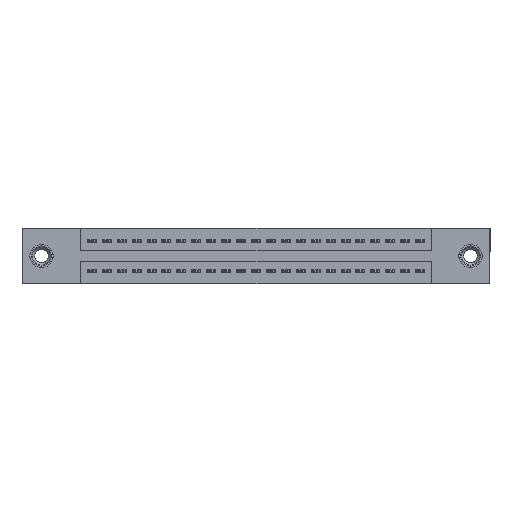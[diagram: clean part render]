
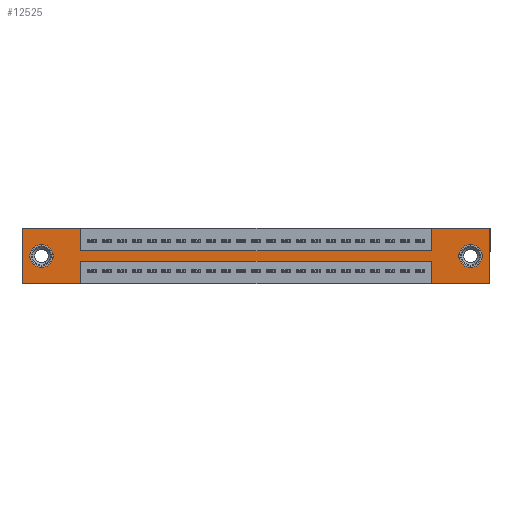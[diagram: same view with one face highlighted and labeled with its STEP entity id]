
A CAD part, front view. The second image highlights one B-rep face of the part: STEP entity #12525.
In plain terms, the highlighted planar face has unit normal (0, -1, 0).
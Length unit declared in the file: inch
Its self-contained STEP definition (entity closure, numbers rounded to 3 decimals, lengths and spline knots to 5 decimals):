
#171 = ORIENTED_EDGE ( 'NONE', *, *, #13784, .F. ) ;
#273 = CARTESIAN_POINT ( 'NONE',  ( 0.13, 0., -0.107 ) ) ;
#340 = ORIENTED_EDGE ( 'NONE', *, *, #17543, .T. ) ;
#410 = EDGE_LOOP ( 'NONE', ( #13257, #13475 ) ) ;
#451 = DIRECTION ( 'NONE',  ( 0., 0., -1. ) ) ;
#464 = EDGE_CURVE ( 'NONE', #20252, #8960, #3851, .T. ) ;
#544 = CARTESIAN_POINT ( 'NONE',  ( 2.7425, 0., -0.22 ) ) ;
#915 = ORIENTED_EDGE ( 'NONE', *, *, #18903, .F. ) ;
#1435 = VERTEX_POINT ( 'NONE', #4557 ) ;
#1554 = CARTESIAN_POINT ( 'NONE',  ( 0.13, 0., -0.185 ) ) ;
#1618 = DIRECTION ( 'NONE',  ( 0., 0., -1. ) ) ;
#1810 = EDGE_CURVE ( 'NONE', #9159, #22244, #9856, .T. ) ;
#1823 = ORIENTED_EDGE ( 'NONE', *, *, #2912, .F. ) ;
#2026 = ORIENTED_EDGE ( 'NONE', *, *, #22330, .F. ) ;
#2217 = CARTESIAN_POINT ( 'NONE',  ( 0.13, 0., -0.185 ) ) ;
#2426 = CARTESIAN_POINT ( 'NONE',  ( 0., 0., 0. ) ) ;
#2560 = EDGE_CURVE ( 'NONE', #12127, #13244, #21114, .T. ) ;
#2655 = VERTEX_POINT ( 'NONE', #544 ) ;
#2698 = CARTESIAN_POINT ( 'NONE',  ( 0.3925, 0., -0.15 ) ) ;
#2912 = EDGE_CURVE ( 'NONE', #1435, #11162, #18052, .T. ) ;
#2942 = VECTOR ( 'NONE', #13759, 39.37008 ) ;
#3134 = ORIENTED_EDGE ( 'NONE', *, *, #1810, .F. ) ;
#3271 = CARTESIAN_POINT ( 'NONE',  ( 3.005, 0., -0.185 ) ) ;
#3345 = DIRECTION ( 'NONE',  ( 0., 1., 0. ) ) ;
#3521 = CARTESIAN_POINT ( 'NONE',  ( 0.3925, 0., -0.22 ) ) ;
#3594 = EDGE_CURVE ( 'NONE', #22244, #1435, #12808, .T. ) ;
#3652 = FACE_BOUND ( 'NONE', #10727, .T. ) ;
#3748 = VERTEX_POINT ( 'NONE', #6160 ) ;
#3851 = CIRCLE ( 'NONE', #9692, 0.078 ) ;
#3881 = CARTESIAN_POINT ( 'NONE',  ( 2.7425, 0., -0.15 ) ) ;
#3914 = ORIENTED_EDGE ( 'NONE', *, *, #2560, .F. ) ;
#4052 = DIRECTION ( 'NONE',  ( 0., 1., 0. ) ) ;
#4064 = EDGE_LOOP ( 'NONE', ( #11508, #171, #2026, #15246, #8780, #3914, #5258, #915, #1823, #7195, #3134, #10701 ) ) ;
#4158 = DIRECTION ( 'NONE',  ( 0., 0., 1. ) ) ;
#4199 = CARTESIAN_POINT ( 'NONE',  ( 0., 0., -0.37 ) ) ;
#4557 = CARTESIAN_POINT ( 'NONE',  ( 0.3925, 0., 0. ) ) ;
#4967 = DIRECTION ( 'NONE',  ( 0., -1., 0. ) ) ;
#5021 = DIRECTION ( 'NONE',  ( 0., 0., -1. ) ) ;
#5258 = ORIENTED_EDGE ( 'NONE', *, *, #8798, .F. ) ;
#5530 = VERTEX_POINT ( 'NONE', #17342 ) ;
#5732 = DIRECTION ( 'NONE',  ( 0., 0., -1. ) ) ;
#6044 = DIRECTION ( 'NONE',  ( 0., 0., -1. ) ) ;
#6121 = CARTESIAN_POINT ( 'NONE',  ( 3.135, 0., 0. ) ) ;
#6160 = CARTESIAN_POINT ( 'NONE',  ( 3.135, 0., -0.37 ) ) ;
#6369 = CIRCLE ( 'NONE', #15278, 0.078 ) ;
#6505 = LINE ( 'NONE', #7549, #13052 ) ;
#7115 = CIRCLE ( 'NONE', #18840, 0.078 ) ;
#7195 = ORIENTED_EDGE ( 'NONE', *, *, #3594, .F. ) ;
#7262 = CARTESIAN_POINT ( 'NONE',  ( 0., 0., 0. ) ) ;
#7311 = DIRECTION ( 'NONE',  ( 0., 1., 0. ) ) ;
#7549 = CARTESIAN_POINT ( 'NONE',  ( 0.3925, 0., -0.15 ) ) ;
#7728 = DIRECTION ( 'NONE',  ( 0., 0., 1. ) ) ;
#8178 = VECTOR ( 'NONE', #21465, 39.37008 ) ;
#8234 = VERTEX_POINT ( 'NONE', #3881 ) ;
#8780 = ORIENTED_EDGE ( 'NONE', *, *, #18987, .F. ) ;
#8798 = EDGE_CURVE ( 'NONE', #8234, #12127, #12153, .T. ) ;
#8960 = VERTEX_POINT ( 'NONE', #20332 ) ;
#9159 = VERTEX_POINT ( 'NONE', #16799 ) ;
#9246 = CARTESIAN_POINT ( 'NONE',  ( 0.3925, 0., -0.37 ) ) ;
#9294 = DIRECTION ( 'NONE',  ( 1., 0., 0. ) ) ;
#9480 = VERTEX_POINT ( 'NONE', #15497 ) ;
#9627 = CARTESIAN_POINT ( 'NONE',  ( 2.7425, 0., 0. ) ) ;
#9692 = AXIS2_PLACEMENT_3D ( 'NONE', #2217, #7311, #21363 ) ;
#9699 = LINE ( 'NONE', #11711, #19200 ) ;
#9804 = EDGE_CURVE ( 'NONE', #18701, #9159, #10468, .T. ) ;
#9856 = LINE ( 'NONE', #11465, #17836 ) ;
#10468 = LINE ( 'NONE', #11045, #20392 ) ;
#10488 = EDGE_CURVE ( 'NONE', #22385, #18701, #17869, .T. ) ;
#10538 = FACE_OUTER_BOUND ( 'NONE', #4064, .T. ) ;
#10561 = FACE_BOUND ( 'NONE', #410, .T. ) ;
#10701 = ORIENTED_EDGE ( 'NONE', *, *, #9804, .F. ) ;
#10727 = EDGE_LOOP ( 'NONE', ( #13237, #340 ) ) ;
#11045 = CARTESIAN_POINT ( 'NONE',  ( 0., 0., -0.37 ) ) ;
#11072 = VECTOR ( 'NONE', #7728, 39.37008 ) ;
#11162 = VERTEX_POINT ( 'NONE', #2698 ) ;
#11170 = DIRECTION ( 'NONE',  ( 1., 0., 0. ) ) ;
#11171 = VECTOR ( 'NONE', #6044, 39.37008 ) ;
#11465 = CARTESIAN_POINT ( 'NONE',  ( 0., 0., 0. ) ) ;
#11508 = ORIENTED_EDGE ( 'NONE', *, *, #10488, .F. ) ;
#11711 = CARTESIAN_POINT ( 'NONE',  ( 2.7425, 0., -0.37 ) ) ;
#12127 = VERTEX_POINT ( 'NONE', #14208 ) ;
#12153 = LINE ( 'NONE', #9627, #11072 ) ;
#12490 = AXIS2_PLACEMENT_3D ( 'NONE', #20826, #4967, #1618 ) ;
#12525 = ADVANCED_FACE ( 'NONE', ( #10561, #3652, #10538 ), #15531, .T. ) ;
#12808 = LINE ( 'NONE', #7262, #8178 ) ;
#12869 = DIRECTION ( 'NONE',  ( -1., 0., 0. ) ) ;
#13052 = VECTOR ( 'NONE', #9294, 39.37008 ) ;
#13113 = EDGE_CURVE ( 'NONE', #20470, #9480, #7115, .T. ) ;
#13181 = VECTOR ( 'NONE', #22395, 39.37008 ) ;
#13237 = ORIENTED_EDGE ( 'NONE', *, *, #464, .T. ) ;
#13244 = VERTEX_POINT ( 'NONE', #6121 ) ;
#13257 = ORIENTED_EDGE ( 'NONE', *, *, #15380, .T. ) ;
#13364 = CARTESIAN_POINT ( 'NONE',  ( 3.135, 0., 0. ) ) ;
#13475 = ORIENTED_EDGE ( 'NONE', *, *, #13113, .T. ) ;
#13759 = DIRECTION ( 'NONE',  ( -1., 0., 0. ) ) ;
#13784 = EDGE_CURVE ( 'NONE', #2655, #22385, #18850, .T. ) ;
#13879 = DIRECTION ( 'NONE',  ( 0., 1., 0. ) ) ;
#14208 = CARTESIAN_POINT ( 'NONE',  ( 2.7425, 0., 0. ) ) ;
#14373 = VECTOR ( 'NONE', #12869, 39.37008 ) ;
#15224 = CARTESIAN_POINT ( 'NONE',  ( 0.3925, 0., -0.37 ) ) ;
#15246 = ORIENTED_EDGE ( 'NONE', *, *, #16338, .F. ) ;
#15278 = AXIS2_PLACEMENT_3D ( 'NONE', #1554, #13879, #20682 ) ;
#15380 = EDGE_CURVE ( 'NONE', #9480, #20470, #22180, .T. ) ;
#15497 = CARTESIAN_POINT ( 'NONE',  ( 3.005, 0., -0.107 ) ) ;
#15531 = PLANE ( 'NONE',  #12490 ) ;
#16338 = EDGE_CURVE ( 'NONE', #3748, #5530, #17690, .T. ) ;
#16449 = DIRECTION ( 'NONE',  ( -1., 0., 0. ) ) ;
#16501 = CARTESIAN_POINT ( 'NONE',  ( 0., 0., 0. ) ) ;
#16799 = CARTESIAN_POINT ( 'NONE',  ( 0., 0., -0.37 ) ) ;
#17268 = VECTOR ( 'NONE', #5732, 39.37008 ) ;
#17342 = CARTESIAN_POINT ( 'NONE',  ( 2.7425, 0., -0.37 ) ) ;
#17543 = EDGE_CURVE ( 'NONE', #8960, #20252, #6369, .T. ) ;
#17690 = LINE ( 'NONE', #4199, #14373 ) ;
#17836 = VECTOR ( 'NONE', #4158, 39.37008 ) ;
#17869 = LINE ( 'NONE', #15224, #13181 ) ;
#17958 = CARTESIAN_POINT ( 'NONE',  ( 3.005, 0., -0.263 ) ) ;
#18052 = LINE ( 'NONE', #20345, #11171 ) ;
#18701 = VERTEX_POINT ( 'NONE', #9246 ) ;
#18840 = AXIS2_PLACEMENT_3D ( 'NONE', #3271, #3345, #5021 ) ;
#18850 = LINE ( 'NONE', #3521, #2942 ) ;
#18896 = LINE ( 'NONE', #13364, #17268 ) ;
#18903 = EDGE_CURVE ( 'NONE', #11162, #8234, #6505, .T. ) ;
#18987 = EDGE_CURVE ( 'NONE', #13244, #3748, #18896, .T. ) ;
#19200 = VECTOR ( 'NONE', #20322, 39.37008 ) ;
#19490 = AXIS2_PLACEMENT_3D ( 'NONE', #19719, #4052, #451 ) ;
#19719 = CARTESIAN_POINT ( 'NONE',  ( 3.005, 0., -0.185 ) ) ;
#20252 = VERTEX_POINT ( 'NONE', #273 ) ;
#20322 = DIRECTION ( 'NONE',  ( 0., 0., 1. ) ) ;
#20332 = CARTESIAN_POINT ( 'NONE',  ( 0.13, 0., -0.263 ) ) ;
#20345 = CARTESIAN_POINT ( 'NONE',  ( 0.3925, 0., 0. ) ) ;
#20392 = VECTOR ( 'NONE', #16449, 39.37008 ) ;
#20470 = VERTEX_POINT ( 'NONE', #17958 ) ;
#20581 = VECTOR ( 'NONE', #11170, 39.37008 ) ;
#20682 = DIRECTION ( 'NONE',  ( 0., 0., 1. ) ) ;
#20826 = CARTESIAN_POINT ( 'NONE',  ( 0., 0., -0.37 ) ) ;
#21114 = LINE ( 'NONE', #16501, #20581 ) ;
#21363 = DIRECTION ( 'NONE',  ( 0., 0., 1. ) ) ;
#21465 = DIRECTION ( 'NONE',  ( 1., 0., 0. ) ) ;
#22180 = CIRCLE ( 'NONE', #19490, 0.078 ) ;
#22206 = CARTESIAN_POINT ( 'NONE',  ( 0.3925, 0., -0.22 ) ) ;
#22244 = VERTEX_POINT ( 'NONE', #2426 ) ;
#22330 = EDGE_CURVE ( 'NONE', #5530, #2655, #9699, .T. ) ;
#22385 = VERTEX_POINT ( 'NONE', #22206 ) ;
#22395 = DIRECTION ( 'NONE',  ( 0., 0., -1. ) ) ;
